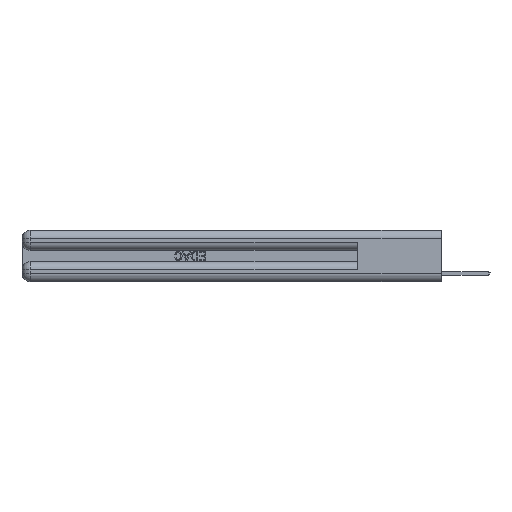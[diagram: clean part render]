
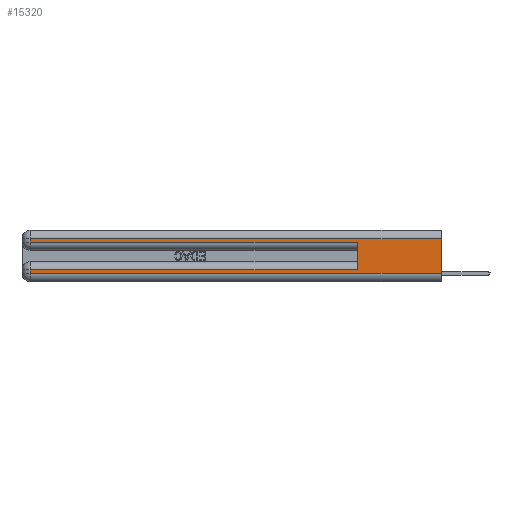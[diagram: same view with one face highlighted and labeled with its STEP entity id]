
A CAD part, left-side view. The second image highlights one B-rep face of the part: STEP entity #15320.
In plain terms, the highlighted planar face has unit normal (-1, 0, 0).
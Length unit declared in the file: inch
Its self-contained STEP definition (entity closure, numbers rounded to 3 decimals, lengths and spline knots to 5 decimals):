
#482 = CARTESIAN_POINT ( 'NONE',  ( 0., 0., 0.31 ) ) ;
#618 = ORIENTED_EDGE ( 'NONE', *, *, #7051, .T. ) ;
#921 = VERTEX_POINT ( 'NONE', #21308 ) ;
#984 = PLANE ( 'NONE',  #10934 ) ;
#1225 = DIRECTION ( 'NONE',  ( 0., 0., -1. ) ) ;
#1324 = CARTESIAN_POINT ( 'NONE',  ( 0., 0., 0.37 ) ) ;
#1363 = LINE ( 'NONE', #23897, #12920 ) ;
#1368 = EDGE_CURVE ( 'NONE', #20337, #27884, #29508, .T. ) ;
#1828 = CARTESIAN_POINT ( 'NONE',  ( 0., 2.94, 0.37 ) ) ;
#2394 = ORIENTED_EDGE ( 'NONE', *, *, #20504, .F. ) ;
#2803 = LINE ( 'NONE', #482, #9263 ) ;
#3881 = LINE ( 'NONE', #23434, #6024 ) ;
#5407 = LINE ( 'NONE', #1324, #14866 ) ;
#5434 = CARTESIAN_POINT ( 'NONE',  ( 0., 2.94, 0.085 ) ) ;
#5958 = CARTESIAN_POINT ( 'NONE',  ( 0., 2.94, 0.31 ) ) ;
#6024 = VECTOR ( 'NONE', #11725, 39.37008 ) ;
#6130 = EDGE_CURVE ( 'NONE', #12066, #14550, #8219, .T. ) ;
#6239 = ORIENTED_EDGE ( 'NONE', *, *, #19680, .T. ) ;
#6269 = CARTESIAN_POINT ( 'NONE',  ( 0., 2.94, 0.37 ) ) ;
#6458 = CARTESIAN_POINT ( 'NONE',  ( 0., 0., 0.06 ) ) ;
#7051 = EDGE_CURVE ( 'NONE', #9325, #12066, #2803, .T. ) ;
#8219 = LINE ( 'NONE', #6269, #27397 ) ;
#8573 = DIRECTION ( 'NONE',  ( 0., 0., -1. ) ) ;
#9050 = DIRECTION ( 'NONE',  ( 0., 0., -1. ) ) ;
#9261 = EDGE_CURVE ( 'NONE', #9325, #27884, #5407, .T. ) ;
#9263 = VECTOR ( 'NONE', #11107, 39.37008 ) ;
#9325 = VERTEX_POINT ( 'NONE', #17688 ) ;
#10169 = VECTOR ( 'NONE', #11986, 39.37008 ) ;
#10364 = CARTESIAN_POINT ( 'NONE',  ( 0., 0.6, 0.285 ) ) ;
#10569 = ORIENTED_EDGE ( 'NONE', *, *, #1368, .T. ) ;
#10934 = AXIS2_PLACEMENT_3D ( 'NONE', #19603, #27025, #24946 ) ;
#11107 = DIRECTION ( 'NONE',  ( 0., 1., 0. ) ) ;
#11725 = DIRECTION ( 'NONE',  ( 0., 0., 1. ) ) ;
#11986 = DIRECTION ( 'NONE',  ( 0., 1., 0. ) ) ;
#12066 = VERTEX_POINT ( 'NONE', #5958 ) ;
#12730 = ORIENTED_EDGE ( 'NONE', *, *, #9261, .F. ) ;
#12920 = VECTOR ( 'NONE', #28444, 39.37008 ) ;
#14491 = ORIENTED_EDGE ( 'NONE', *, *, #6130, .T. ) ;
#14550 = VERTEX_POINT ( 'NONE', #26811 ) ;
#14866 = VECTOR ( 'NONE', #1225, 39.37008 ) ;
#15320 = ADVANCED_FACE ( 'NONE', ( #18721 ), #984, .F. ) ;
#17107 = EDGE_LOOP ( 'NONE', ( #12730, #618, #14491, #6239, #2394, #17248, #28151, #10569 ) ) ;
#17248 = ORIENTED_EDGE ( 'NONE', *, *, #17329, .T. ) ;
#17329 = EDGE_CURVE ( 'NONE', #921, #18445, #20068, .T. ) ;
#17493 = CARTESIAN_POINT ( 'NONE',  ( 0., 2.94, 0.06 ) ) ;
#17688 = CARTESIAN_POINT ( 'NONE',  ( 0., 0., 0.31 ) ) ;
#18006 = VECTOR ( 'NONE', #9050, 39.37008 ) ;
#18445 = VERTEX_POINT ( 'NONE', #5434 ) ;
#18721 = FACE_OUTER_BOUND ( 'NONE', #17107, .T. ) ;
#19603 = CARTESIAN_POINT ( 'NONE',  ( 0., 0., 0.37 ) ) ;
#19680 = EDGE_CURVE ( 'NONE', #14550, #30034, #1363, .T. ) ;
#20068 = LINE ( 'NONE', #21421, #10169 ) ;
#20337 = VERTEX_POINT ( 'NONE', #17493 ) ;
#20504 = EDGE_CURVE ( 'NONE', #921, #30034, #3881, .T. ) ;
#21308 = CARTESIAN_POINT ( 'NONE',  ( 0., 0.6, 0.085 ) ) ;
#21421 = CARTESIAN_POINT ( 'NONE',  ( 0., 0., 0.085 ) ) ;
#22844 = DIRECTION ( 'NONE',  ( 0., -1., 0. ) ) ;
#23019 = EDGE_CURVE ( 'NONE', #18445, #20337, #28735, .T. ) ;
#23434 = CARTESIAN_POINT ( 'NONE',  ( 0., 0.6, 0.145 ) ) ;
#23897 = CARTESIAN_POINT ( 'NONE',  ( 0., 0., 0.285 ) ) ;
#24946 = DIRECTION ( 'NONE',  ( 0., 0., -1. ) ) ;
#26811 = CARTESIAN_POINT ( 'NONE',  ( 0., 2.94, 0.285 ) ) ;
#27025 = DIRECTION ( 'NONE',  ( 1., 0., 0. ) ) ;
#27303 = VECTOR ( 'NONE', #22844, 39.37008 ) ;
#27397 = VECTOR ( 'NONE', #8573, 39.37008 ) ;
#27884 = VERTEX_POINT ( 'NONE', #29632 ) ;
#28151 = ORIENTED_EDGE ( 'NONE', *, *, #23019, .T. ) ;
#28444 = DIRECTION ( 'NONE',  ( 0., -1., 0. ) ) ;
#28735 = LINE ( 'NONE', #1828, #18006 ) ;
#29508 = LINE ( 'NONE', #6458, #27303 ) ;
#29632 = CARTESIAN_POINT ( 'NONE',  ( 0., 0., 0.06 ) ) ;
#30034 = VERTEX_POINT ( 'NONE', #10364 ) ;
